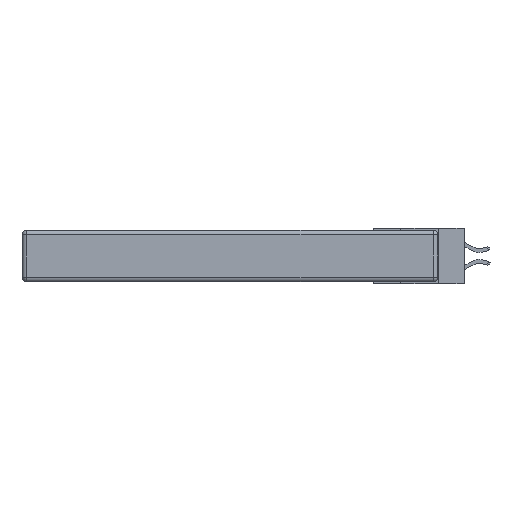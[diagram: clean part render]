
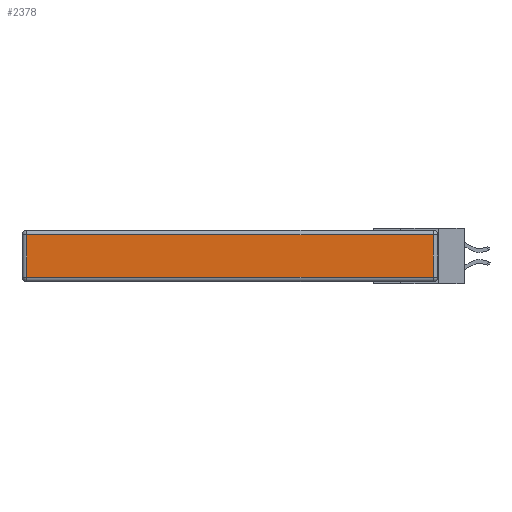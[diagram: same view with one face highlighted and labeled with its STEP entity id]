
A CAD part, left-side view. The second image highlights one B-rep face of the part: STEP entity #2378.
In plain terms, the highlighted planar face has unit normal (-1, 0, 0).
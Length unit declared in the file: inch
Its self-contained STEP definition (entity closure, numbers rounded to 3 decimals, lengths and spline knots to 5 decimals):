
#2378 = ADVANCED_FACE ( 'NONE', ( #24591 ), #25448, .T. ) ;
#3163 = AXIS2_PLACEMENT_3D ( 'NONE', #18162, #20583, #11414 ) ;
#4318 = EDGE_CURVE ( 'NONE', #13885, #29997, #16518, .T. ) ;
#4955 = ORIENTED_EDGE ( 'NONE', *, *, #17061, .T. ) ;
#5541 = DIRECTION ( 'NONE',  ( 0., 1., 0. ) ) ;
#5638 = DIRECTION ( 'NONE',  ( 0., 0., 1. ) ) ;
#5844 = LINE ( 'NONE', #17834, #29227 ) ;
#9232 = ORIENTED_EDGE ( 'NONE', *, *, #25503, .T. ) ;
#9799 = LINE ( 'NONE', #24084, #23371 ) ;
#10114 = VECTOR ( 'NONE', #5541, 39.37008 ) ;
#10868 = DIRECTION ( 'NONE',  ( 0., -1., 0. ) ) ;
#11414 = DIRECTION ( 'NONE',  ( 0., 0., 1. ) ) ;
#13885 = VERTEX_POINT ( 'NONE', #24321 ) ;
#14163 = EDGE_CURVE ( 'NONE', #29997, #29225, #9799, .T. ) ;
#15202 = VERTEX_POINT ( 'NONE', #27431 ) ;
#15397 = ORIENTED_EDGE ( 'NONE', *, *, #4318, .T. ) ;
#15437 = EDGE_LOOP ( 'NONE', ( #4955, #9232, #15397, #27432 ) ) ;
#16518 = LINE ( 'NONE', #21903, #10114 ) ;
#17061 = EDGE_CURVE ( 'NONE', #29225, #15202, #5844, .T. ) ;
#17834 = CARTESIAN_POINT ( 'NONE',  ( 0., 0., -0.313 ) ) ;
#18162 = CARTESIAN_POINT ( 'NONE',  ( 0., 0., -0.343 ) ) ;
#19308 = DIRECTION ( 'NONE',  ( 0., 0., -1. ) ) ;
#19858 = CARTESIAN_POINT ( 'NONE',  ( 0., 0.03, -0.343 ) ) ;
#20583 = DIRECTION ( 'NONE',  ( -1., 0., 0. ) ) ;
#21897 = CARTESIAN_POINT ( 'NONE',  ( 0., 2.72, -0.03 ) ) ;
#21903 = CARTESIAN_POINT ( 'NONE',  ( 0., 2.75, -0.03 ) ) ;
#23371 = VECTOR ( 'NONE', #19308, 39.37008 ) ;
#23387 = VECTOR ( 'NONE', #5638, 39.37008 ) ;
#24084 = CARTESIAN_POINT ( 'NONE',  ( 0., 2.72, -0.343 ) ) ;
#24321 = CARTESIAN_POINT ( 'NONE',  ( 0., 0.03, -0.03 ) ) ;
#24591 = FACE_OUTER_BOUND ( 'NONE', #15437, .T. ) ;
#25448 = PLANE ( 'NONE',  #3163 ) ;
#25503 = EDGE_CURVE ( 'NONE', #15202, #13885, #30511, .T. ) ;
#26171 = CARTESIAN_POINT ( 'NONE',  ( 0., 2.72, -0.313 ) ) ;
#27431 = CARTESIAN_POINT ( 'NONE',  ( 0., 0.03, -0.313 ) ) ;
#27432 = ORIENTED_EDGE ( 'NONE', *, *, #14163, .T. ) ;
#29225 = VERTEX_POINT ( 'NONE', #26171 ) ;
#29227 = VECTOR ( 'NONE', #10868, 39.37008 ) ;
#29997 = VERTEX_POINT ( 'NONE', #21897 ) ;
#30511 = LINE ( 'NONE', #19858, #23387 ) ;
